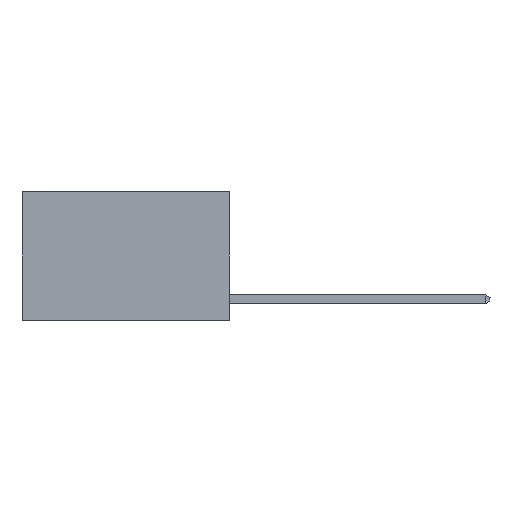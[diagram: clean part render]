
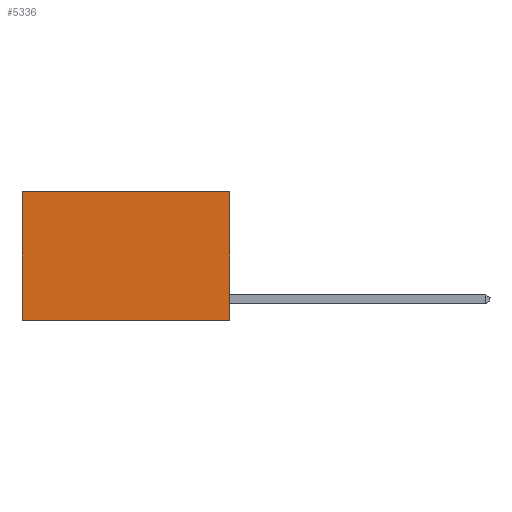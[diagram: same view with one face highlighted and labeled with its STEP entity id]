
A CAD part, left-side view. The second image highlights one B-rep face of the part: STEP entity #5336.
In plain terms, the highlighted planar face has unit normal (-1, 0, 0).
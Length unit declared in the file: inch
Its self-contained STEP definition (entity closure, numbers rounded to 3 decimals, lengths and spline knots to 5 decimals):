
#307 = LINE ( 'NONE', #16943, #2586 ) ;
#1068 = DIRECTION ( 'NONE',  ( 0., 1., 0. ) ) ;
#1510 = CARTESIAN_POINT ( 'NONE',  ( 0.2625, 0., 0. ) ) ;
#1679 = LINE ( 'NONE', #14833, #18571 ) ;
#2586 = VECTOR ( 'NONE', #25801, 39.37008 ) ;
#2800 = EDGE_CURVE ( 'NONE', #19608, #17940, #10077, .T. ) ;
#3207 = DIRECTION ( 'NONE',  ( 0., 0., -1. ) ) ;
#3791 = DIRECTION ( 'NONE',  ( 0., 1., 0. ) ) ;
#4613 = VERTEX_POINT ( 'NONE', #23725 ) ;
#5336 = ADVANCED_FACE ( 'NONE', ( #11806 ), #26816, .F. ) ;
#5487 = EDGE_CURVE ( 'NONE', #4613, #17940, #307, .T. ) ;
#7210 = DIRECTION ( 'NONE',  ( 1., 0., 0. ) ) ;
#9259 = CARTESIAN_POINT ( 'NONE',  ( 0.2625, 0.6, -0.37 ) ) ;
#9903 = AXIS2_PLACEMENT_3D ( 'NONE', #22670, #7210, #3207 ) ;
#10077 = LINE ( 'NONE', #16107, #23759 ) ;
#10503 = ORIENTED_EDGE ( 'NONE', *, *, #5487, .T. ) ;
#10581 = ORIENTED_EDGE ( 'NONE', *, *, #18244, .F. ) ;
#11806 = FACE_OUTER_BOUND ( 'NONE', #12218, .T. ) ;
#12218 = EDGE_LOOP ( 'NONE', ( #10503, #20238, #10581, #26034 ) ) ;
#12239 = LINE ( 'NONE', #1510, #25322 ) ;
#14833 = CARTESIAN_POINT ( 'NONE',  ( 0.2625, 0., 0. ) ) ;
#14990 = EDGE_CURVE ( 'NONE', #25823, #4613, #12239, .T. ) ;
#16107 = CARTESIAN_POINT ( 'NONE',  ( 0.2625, 0., -0.37 ) ) ;
#16943 = CARTESIAN_POINT ( 'NONE',  ( 0.2625, 0.6, 0. ) ) ;
#17940 = VERTEX_POINT ( 'NONE', #9259 ) ;
#18244 = EDGE_CURVE ( 'NONE', #25823, #19608, #1679, .T. ) ;
#18571 = VECTOR ( 'NONE', #27552, 39.37008 ) ;
#19608 = VERTEX_POINT ( 'NONE', #25075 ) ;
#20238 = ORIENTED_EDGE ( 'NONE', *, *, #2800, .F. ) ;
#22670 = CARTESIAN_POINT ( 'NONE',  ( 0.2625, 0., 0. ) ) ;
#23650 = CARTESIAN_POINT ( 'NONE',  ( 0.2625, 0., 0. ) ) ;
#23725 = CARTESIAN_POINT ( 'NONE',  ( 0.2625, 0.6, 0. ) ) ;
#23759 = VECTOR ( 'NONE', #1068, 39.37008 ) ;
#25075 = CARTESIAN_POINT ( 'NONE',  ( 0.2625, 0., -0.37 ) ) ;
#25322 = VECTOR ( 'NONE', #3791, 39.37008 ) ;
#25801 = DIRECTION ( 'NONE',  ( 0., 0., -1. ) ) ;
#25823 = VERTEX_POINT ( 'NONE', #23650 ) ;
#26034 = ORIENTED_EDGE ( 'NONE', *, *, #14990, .T. ) ;
#26816 = PLANE ( 'NONE',  #9903 ) ;
#27552 = DIRECTION ( 'NONE',  ( 0., 0., -1. ) ) ;
